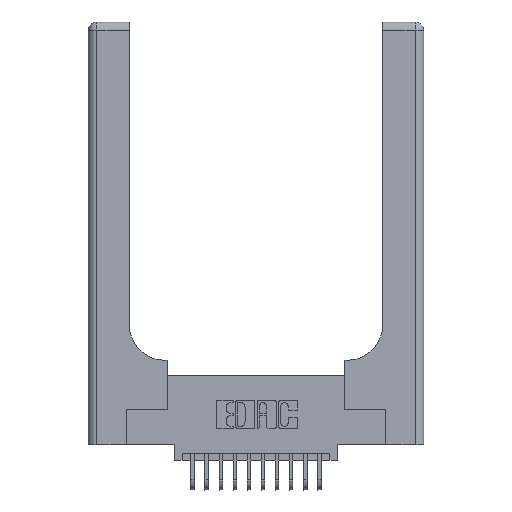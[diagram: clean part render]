
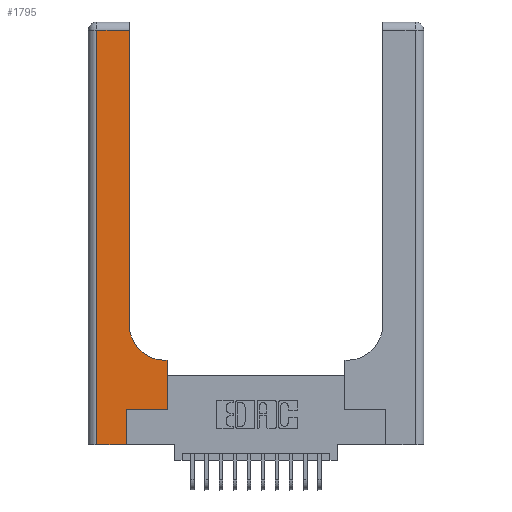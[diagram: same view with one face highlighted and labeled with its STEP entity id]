
A CAD part, top view. The second image highlights one B-rep face of the part: STEP entity #1795.
In plain terms, the highlighted planar face has unit normal (0, 0, 1).
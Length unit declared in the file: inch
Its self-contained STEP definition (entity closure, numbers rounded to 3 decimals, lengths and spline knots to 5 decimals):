
#58 = CARTESIAN_POINT ( 'NONE',  ( 0., 3., 0.37 ) ) ;
#81 = DIRECTION ( 'NONE',  ( 1., 0., 0. ) ) ;
#122 = VERTEX_POINT ( 'NONE', #16376 ) ;
#318 = VECTOR ( 'NONE', #5777, 39.37008 ) ;
#730 = CARTESIAN_POINT ( 'NONE',  ( 0.2915, 0.85, 0.37 ) ) ;
#1051 = ORIENTED_EDGE ( 'NONE', *, *, #1308, .T. ) ;
#1232 = VECTOR ( 'NONE', #1569, 39.37008 ) ;
#1308 = EDGE_CURVE ( 'NONE', #3528, #2310, #12476, .T. ) ;
#1327 = PLANE ( 'NONE',  #8361 ) ;
#1368 = ORIENTED_EDGE ( 'NONE', *, *, #7239, .T. ) ;
#1463 = ORIENTED_EDGE ( 'NONE', *, *, #17689, .T. ) ;
#1569 = DIRECTION ( 'NONE',  ( -1., 0., 0. ) ) ;
#1643 = CARTESIAN_POINT ( 'NONE',  ( 0.5415, 0.6, 0.37 ) ) ;
#1768 = ORIENTED_EDGE ( 'NONE', *, *, #9782, .T. ) ;
#1795 = ADVANCED_FACE ( 'NONE', ( #10874 ), #1327, .F. ) ;
#1969 = CARTESIAN_POINT ( 'NONE',  ( 0.269, 0.25, 0.37 ) ) ;
#2000 = CARTESIAN_POINT ( 'NONE',  ( 0.5585, 0.6, 0.37 ) ) ;
#2310 = VERTEX_POINT ( 'NONE', #1643 ) ;
#2329 = CARTESIAN_POINT ( 'NONE',  ( 0.5415, 0.85, 0.37 ) ) ;
#2432 = CARTESIAN_POINT ( 'NONE',  ( 0.2915, 0.6, 0.37 ) ) ;
#3435 = EDGE_CURVE ( 'NONE', #6761, #122, #7569, .T. ) ;
#3528 = VERTEX_POINT ( 'NONE', #2000 ) ;
#3545 = DIRECTION ( 'NONE',  ( 0., 1., 0. ) ) ;
#3765 = DIRECTION ( 'NONE',  ( 0., 0., -1. ) ) ;
#4424 = CARTESIAN_POINT ( 'NONE',  ( 0.06, 0., 0.37 ) ) ;
#4518 = EDGE_LOOP ( 'NONE', ( #16697, #11720, #14386, #17090, #1368, #1768, #8956, #1051, #1463 ) ) ;
#4922 = CARTESIAN_POINT ( 'NONE',  ( 0.2915, 3., 0.37 ) ) ;
#5777 = DIRECTION ( 'NONE',  ( 0., -1., 0. ) ) ;
#5793 = DIRECTION ( 'NONE',  ( 0., 0., -1. ) ) ;
#5935 = VECTOR ( 'NONE', #12322, 39.37008 ) ;
#6332 = LINE ( 'NONE', #7919, #16973 ) ;
#6461 = CARTESIAN_POINT ( 'NONE',  ( 0.2915, 2.94, 0.37 ) ) ;
#6761 = VERTEX_POINT ( 'NONE', #4424 ) ;
#7209 = DIRECTION ( 'NONE',  ( -1., 0., 0. ) ) ;
#7239 = EDGE_CURVE ( 'NONE', #122, #9854, #9654, .T. ) ;
#7569 = LINE ( 'NONE', #17945, #12625 ) ;
#7919 = CARTESIAN_POINT ( 'NONE',  ( 0.5585, 0.25, 0.37 ) ) ;
#8361 = AXIS2_PLACEMENT_3D ( 'NONE', #58, #5793, #7209 ) ;
#8532 = AXIS2_PLACEMENT_3D ( 'NONE', #2329, #3765, #11208 ) ;
#8670 = CARTESIAN_POINT ( 'NONE',  ( 0.06, 3., 0.37 ) ) ;
#8921 = CARTESIAN_POINT ( 'NONE',  ( 0.269, 0.25, 0.37 ) ) ;
#8956 = ORIENTED_EDGE ( 'NONE', *, *, #9216, .T. ) ;
#9102 = LINE ( 'NONE', #14828, #1232 ) ;
#9216 = EDGE_CURVE ( 'NONE', #16672, #3528, #6332, .T. ) ;
#9654 = LINE ( 'NONE', #10853, #5935 ) ;
#9782 = EDGE_CURVE ( 'NONE', #9854, #16672, #15336, .T. ) ;
#9854 = VERTEX_POINT ( 'NONE', #1969 ) ;
#9951 = CARTESIAN_POINT ( 'NONE',  ( 0.5585, 0.25, 0.37 ) ) ;
#10149 = EDGE_CURVE ( 'NONE', #14579, #16706, #9102, .T. ) ;
#10594 = DIRECTION ( 'NONE',  ( 1., 0., 0. ) ) ;
#10611 = VECTOR ( 'NONE', #3545, 39.37008 ) ;
#10767 = EDGE_CURVE ( 'NONE', #16706, #6761, #15551, .T. ) ;
#10853 = CARTESIAN_POINT ( 'NONE',  ( 0.269, 0., 0.37 ) ) ;
#10874 = FACE_OUTER_BOUND ( 'NONE', #4518, .T. ) ;
#11208 = DIRECTION ( 'NONE',  ( 1., 0., 0. ) ) ;
#11720 = ORIENTED_EDGE ( 'NONE', *, *, #10149, .T. ) ;
#12221 = LINE ( 'NONE', #4922, #10611 ) ;
#12309 = DIRECTION ( 'NONE',  ( 0., 1., 0. ) ) ;
#12322 = DIRECTION ( 'NONE',  ( 0., 1., 0. ) ) ;
#12476 = LINE ( 'NONE', #2432, #15499 ) ;
#12625 = VECTOR ( 'NONE', #10594, 39.37008 ) ;
#13522 = CIRCLE ( 'NONE', #8532, 0.25 ) ;
#14386 = ORIENTED_EDGE ( 'NONE', *, *, #10767, .T. ) ;
#14579 = VERTEX_POINT ( 'NONE', #6461 ) ;
#14828 = CARTESIAN_POINT ( 'NONE',  ( 0., 2.94, 0.37 ) ) ;
#15266 = EDGE_CURVE ( 'NONE', #16596, #14579, #12221, .T. ) ;
#15336 = LINE ( 'NONE', #8921, #17170 ) ;
#15499 = VECTOR ( 'NONE', #15741, 39.37008 ) ;
#15551 = LINE ( 'NONE', #8670, #318 ) ;
#15694 = CARTESIAN_POINT ( 'NONE',  ( 0.06, 2.94, 0.37 ) ) ;
#15741 = DIRECTION ( 'NONE',  ( -1., 0., 0. ) ) ;
#16376 = CARTESIAN_POINT ( 'NONE',  ( 0.269, 0., 0.37 ) ) ;
#16596 = VERTEX_POINT ( 'NONE', #730 ) ;
#16672 = VERTEX_POINT ( 'NONE', #9951 ) ;
#16697 = ORIENTED_EDGE ( 'NONE', *, *, #15266, .T. ) ;
#16706 = VERTEX_POINT ( 'NONE', #15694 ) ;
#16973 = VECTOR ( 'NONE', #12309, 39.37008 ) ;
#17090 = ORIENTED_EDGE ( 'NONE', *, *, #3435, .T. ) ;
#17170 = VECTOR ( 'NONE', #81, 39.37008 ) ;
#17689 = EDGE_CURVE ( 'NONE', #2310, #16596, #13522, .T. ) ;
#17945 = CARTESIAN_POINT ( 'NONE',  ( 0., 0., 0.37 ) ) ;
